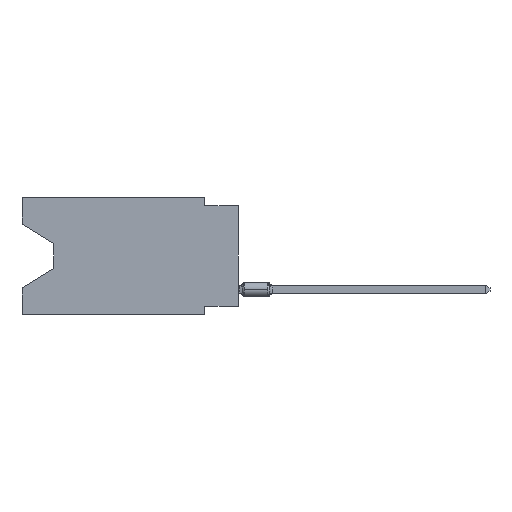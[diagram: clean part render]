
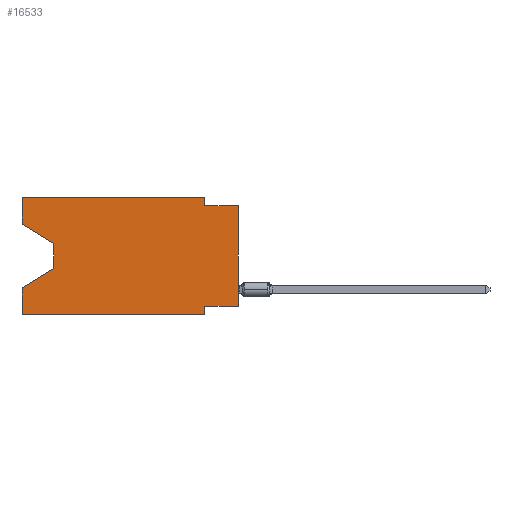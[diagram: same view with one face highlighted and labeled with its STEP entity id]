
A CAD part, left-side view. The second image highlights one B-rep face of the part: STEP entity #16533.
In plain terms, the highlighted planar face has unit normal (-1, 0, 0).
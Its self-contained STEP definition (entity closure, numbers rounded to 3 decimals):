
#21 = ORIENTED_EDGE ( 'NONE', *, *, #18471, .T. ) ;
#239 = EDGE_CURVE ( 'NONE', #17419, #17485, #10327, .T. ) ;
#475 = LINE ( 'NONE', #16055, #8734 ) ;
#914 = EDGE_CURVE ( 'NONE', #22802, #19554, #14364, .T. ) ;
#1494 = CARTESIAN_POINT ( 'NONE',  ( 0., 0., 0. ) ) ;
#1859 = VERTEX_POINT ( 'NONE', #24728 ) ;
#2328 = DIRECTION ( 'NONE',  ( 0., 0., -1. ) ) ;
#2336 = CARTESIAN_POINT ( 'NONE',  ( 0., 13.97, -3.505 ) ) ;
#2458 = LINE ( 'NONE', #2336, #13139 ) ;
#2590 = ORIENTED_EDGE ( 'NONE', *, *, #13669, .T. ) ;
#2779 = LINE ( 'NONE', #13363, #13468 ) ;
#3409 = CARTESIAN_POINT ( 'NONE',  ( 0., 0., -0.635 ) ) ;
#3688 = ORIENTED_EDGE ( 'NONE', *, *, #914, .F. ) ;
#3892 = ORIENTED_EDGE ( 'NONE', *, *, #9755, .F. ) ;
#4025 = VERTEX_POINT ( 'NONE', #7190 ) ;
#4258 = LINE ( 'NONE', #6063, #13100 ) ;
#4596 = EDGE_CURVE ( 'NONE', #1859, #4025, #11822, .T. ) ;
#5256 = VERTEX_POINT ( 'NONE', #6897 ) ;
#5370 = CARTESIAN_POINT ( 'NONE',  ( 0., 16.383, -8.89 ) ) ;
#5450 = DIRECTION ( 'NONE',  ( 0., -1., 0. ) ) ;
#5713 = VECTOR ( 'NONE', #15194, 1000. ) ;
#5834 = CARTESIAN_POINT ( 'NONE',  ( 0., 0., -0.635 ) ) ;
#5846 = VECTOR ( 'NONE', #5450, 1000. ) ;
#6044 = EDGE_CURVE ( 'NONE', #6085, #24020, #2458, .T. ) ;
#6063 = CARTESIAN_POINT ( 'NONE',  ( 0., 2.54, -8.89 ) ) ;
#6085 = VERTEX_POINT ( 'NONE', #12229 ) ;
#6179 = EDGE_CURVE ( 'NONE', #4025, #21696, #4258, .T. ) ;
#6575 = VECTOR ( 'NONE', #22032, 1000. ) ;
#6662 = CARTESIAN_POINT ( 'NONE',  ( 0., 16.383, 0. ) ) ;
#6854 = EDGE_CURVE ( 'NONE', #1859, #20405, #13586, .T. ) ;
#6897 = CARTESIAN_POINT ( 'NONE',  ( 0., 16.383, -6.852 ) ) ;
#6999 = VECTOR ( 'NONE', #8600, 1000. ) ;
#7182 = CARTESIAN_POINT ( 'NONE',  ( 0., 16.383, -2.038 ) ) ;
#7190 = CARTESIAN_POINT ( 'NONE',  ( 0., 2.54, -8.255 ) ) ;
#7417 = VECTOR ( 'NONE', #13758, 1000. ) ;
#8034 = CARTESIAN_POINT ( 'NONE',  ( 0., 2.54, -8.89 ) ) ;
#8055 = EDGE_CURVE ( 'NONE', #16421, #5256, #19077, .T. ) ;
#8103 = CARTESIAN_POINT ( 'NONE',  ( 0., 0., -8.255 ) ) ;
#8251 = ORIENTED_EDGE ( 'NONE', *, *, #6854, .T. ) ;
#8600 = DIRECTION ( 'NONE',  ( 0., -1., 0. ) ) ;
#8734 = VECTOR ( 'NONE', #13988, 1000. ) ;
#9755 = EDGE_CURVE ( 'NONE', #17485, #22802, #15009, .T. ) ;
#10252 = PLANE ( 'NONE',  #15392 ) ;
#10327 = LINE ( 'NONE', #22541, #6575 ) ;
#10432 = ORIENTED_EDGE ( 'NONE', *, *, #6179, .F. ) ;
#10560 = ORIENTED_EDGE ( 'NONE', *, *, #6044, .T. ) ;
#10712 = VECTOR ( 'NONE', #24282, 1000. ) ;
#11746 = ORIENTED_EDGE ( 'NONE', *, *, #11784, .F. ) ;
#11784 = EDGE_CURVE ( 'NONE', #19554, #20405, #21146, .T. ) ;
#11822 = LINE ( 'NONE', #8103, #7417 ) ;
#11954 = EDGE_CURVE ( 'NONE', #17419, #6085, #475, .T. ) ;
#12174 = FACE_OUTER_BOUND ( 'NONE', #24205, .T. ) ;
#12229 = CARTESIAN_POINT ( 'NONE',  ( 0., 13.97, -3.505 ) ) ;
#12479 = ORIENTED_EDGE ( 'NONE', *, *, #8055, .F. ) ;
#13100 = VECTOR ( 'NONE', #2328, 1000. ) ;
#13139 = VECTOR ( 'NONE', #15853, 1000. ) ;
#13185 = ORIENTED_EDGE ( 'NONE', *, *, #11954, .T. ) ;
#13212 = CARTESIAN_POINT ( 'NONE',  ( 0., 2.54, 0. ) ) ;
#13363 = CARTESIAN_POINT ( 'NONE',  ( 0., 16.383, -8.89 ) ) ;
#13468 = VECTOR ( 'NONE', #19672, 1000. ) ;
#13586 = LINE ( 'NONE', #1494, #22695 ) ;
#13669 = EDGE_CURVE ( 'NONE', #16421, #21696, #2779, .T. ) ;
#13758 = DIRECTION ( 'NONE',  ( 0., 1., 0. ) ) ;
#13988 = DIRECTION ( 'NONE',  ( 0., -0.855, -0.519 ) ) ;
#14364 = LINE ( 'NONE', #22092, #10712 ) ;
#15009 = LINE ( 'NONE', #6662, #6999 ) ;
#15194 = DIRECTION ( 'NONE',  ( 0., 0., 1. ) ) ;
#15392 = AXIS2_PLACEMENT_3D ( 'NONE', #17984, #21701, #21963 ) ;
#15636 = ORIENTED_EDGE ( 'NONE', *, *, #239, .F. ) ;
#15853 = DIRECTION ( 'NONE',  ( 0., 0., -1. ) ) ;
#15879 = VECTOR ( 'NONE', #21902, 1000. ) ;
#16055 = CARTESIAN_POINT ( 'NONE',  ( 0., 16.383, -2.038 ) ) ;
#16421 = VERTEX_POINT ( 'NONE', #5370 ) ;
#16533 = ADVANCED_FACE ( 'NONE', ( #12174 ), #10252, .F. ) ;
#17419 = VERTEX_POINT ( 'NONE', #7182 ) ;
#17485 = VERTEX_POINT ( 'NONE', #18526 ) ;
#17984 = CARTESIAN_POINT ( 'NONE',  ( 0., 16.383, 0. ) ) ;
#18055 = CARTESIAN_POINT ( 'NONE',  ( 0., 13.97, -5.385 ) ) ;
#18471 = EDGE_CURVE ( 'NONE', #24020, #5256, #19723, .T. ) ;
#18526 = CARTESIAN_POINT ( 'NONE',  ( 0., 16.383, 0. ) ) ;
#19077 = LINE ( 'NONE', #24984, #5713 ) ;
#19554 = VERTEX_POINT ( 'NONE', #23012 ) ;
#19672 = DIRECTION ( 'NONE',  ( 0., -1., 0. ) ) ;
#19723 = LINE ( 'NONE', #19972, #15879 ) ;
#19972 = CARTESIAN_POINT ( 'NONE',  ( 0., 13.97, -5.385 ) ) ;
#20405 = VERTEX_POINT ( 'NONE', #3409 ) ;
#21062 = DIRECTION ( 'NONE',  ( 0., 0., 1. ) ) ;
#21146 = LINE ( 'NONE', #5834, #5846 ) ;
#21696 = VERTEX_POINT ( 'NONE', #8034 ) ;
#21701 = DIRECTION ( 'NONE',  ( 1., 0., 0. ) ) ;
#21902 = DIRECTION ( 'NONE',  ( 0., 0.855, -0.519 ) ) ;
#21963 = DIRECTION ( 'NONE',  ( 0., 0., -1. ) ) ;
#22032 = DIRECTION ( 'NONE',  ( 0., 0., 1. ) ) ;
#22092 = CARTESIAN_POINT ( 'NONE',  ( 0., 2.54, 0. ) ) ;
#22541 = CARTESIAN_POINT ( 'NONE',  ( 0., 16.383, 0. ) ) ;
#22695 = VECTOR ( 'NONE', #21062, 1000. ) ;
#22802 = VERTEX_POINT ( 'NONE', #13212 ) ;
#23012 = CARTESIAN_POINT ( 'NONE',  ( 0., 2.54, -0.635 ) ) ;
#24020 = VERTEX_POINT ( 'NONE', #18055 ) ;
#24205 = EDGE_LOOP ( 'NONE', ( #13185, #10560, #21, #12479, #2590, #10432, #24208, #8251, #11746, #3688, #3892, #15636 ) ) ;
#24208 = ORIENTED_EDGE ( 'NONE', *, *, #4596, .F. ) ;
#24282 = DIRECTION ( 'NONE',  ( 0., 0., -1. ) ) ;
#24728 = CARTESIAN_POINT ( 'NONE',  ( 0., 0., -8.255 ) ) ;
#24984 = CARTESIAN_POINT ( 'NONE',  ( 0., 16.383, 0. ) ) ;
